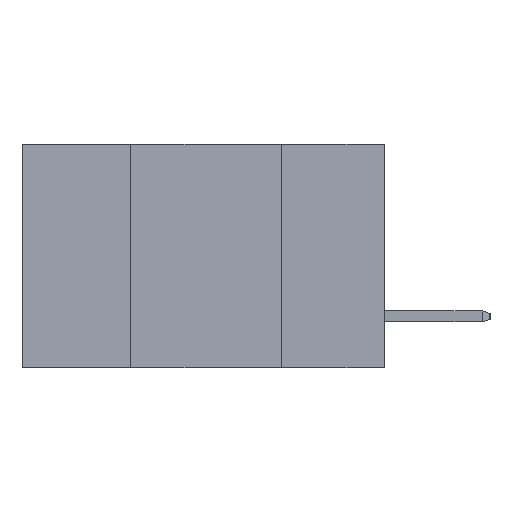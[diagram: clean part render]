
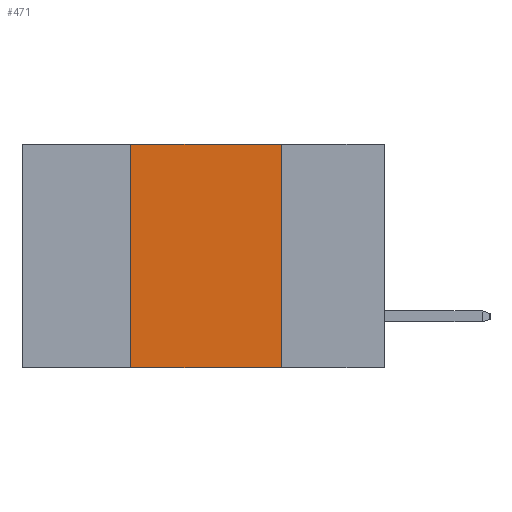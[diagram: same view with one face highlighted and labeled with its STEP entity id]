
A CAD part, left-side view. The second image highlights one B-rep face of the part: STEP entity #471.
In plain terms, the highlighted planar face has unit normal (-1, 0, 0).
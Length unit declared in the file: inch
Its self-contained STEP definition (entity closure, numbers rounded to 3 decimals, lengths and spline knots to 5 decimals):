
#471 = ADVANCED_FACE ( 'NONE', ( #11316 ), #24285, .F. ) ;
#1802 = DIRECTION ( 'NONE',  ( 0., 0., -1. ) ) ;
#3424 = CARTESIAN_POINT ( 'NONE',  ( 0., 0.42, -0.37 ) ) ;
#3860 = CARTESIAN_POINT ( 'NONE',  ( 0., 0.17, 0. ) ) ;
#3966 = DIRECTION ( 'NONE',  ( 0., -1., 0. ) ) ;
#5095 = LINE ( 'NONE', #14805, #22278 ) ;
#5142 = ORIENTED_EDGE ( 'NONE', *, *, #10030, .F. ) ;
#5227 = EDGE_CURVE ( 'NONE', #5744, #25978, #26703, .T. ) ;
#5744 = VERTEX_POINT ( 'NONE', #3860 ) ;
#6261 = CARTESIAN_POINT ( 'NONE',  ( 0., 0.6, 0. ) ) ;
#7250 = ORIENTED_EDGE ( 'NONE', *, *, #17440, .T. ) ;
#9217 = CARTESIAN_POINT ( 'NONE',  ( 0., 0.17, 0. ) ) ;
#10030 = EDGE_CURVE ( 'NONE', #25323, #18070, #23698, .T. ) ;
#10309 = DIRECTION ( 'NONE',  ( 0., -1., 0. ) ) ;
#10807 = CARTESIAN_POINT ( 'NONE',  ( 0., 0.6, 0. ) ) ;
#10934 = EDGE_CURVE ( 'NONE', #18070, #5744, #23215, .T. ) ;
#11316 = FACE_OUTER_BOUND ( 'NONE', #27347, .T. ) ;
#11336 = VECTOR ( 'NONE', #3966, 39.37008 ) ;
#11827 = VECTOR ( 'NONE', #21072, 39.37008 ) ;
#12388 = CARTESIAN_POINT ( 'NONE',  ( 0., 0.17, -0.37 ) ) ;
#13743 = DIRECTION ( 'NONE',  ( 0., 0., -1. ) ) ;
#14102 = DIRECTION ( 'NONE',  ( 1., 0., 0. ) ) ;
#14805 = CARTESIAN_POINT ( 'NONE',  ( 0., 0.6, -0.37 ) ) ;
#16592 = CARTESIAN_POINT ( 'NONE',  ( 0., 0.42, 0. ) ) ;
#17440 = EDGE_CURVE ( 'NONE', #25323, #25978, #5095, .T. ) ;
#18070 = VERTEX_POINT ( 'NONE', #18949 ) ;
#18949 = CARTESIAN_POINT ( 'NONE',  ( 0., 0.42, 0. ) ) ;
#19817 = ORIENTED_EDGE ( 'NONE', *, *, #5227, .F. ) ;
#20820 = VECTOR ( 'NONE', #13743, 39.37008 ) ;
#21072 = DIRECTION ( 'NONE',  ( 0., 0., 1. ) ) ;
#22278 = VECTOR ( 'NONE', #10309, 39.37008 ) ;
#23215 = LINE ( 'NONE', #6261, #11336 ) ;
#23698 = LINE ( 'NONE', #16592, #11827 ) ;
#24048 = ORIENTED_EDGE ( 'NONE', *, *, #10934, .F. ) ;
#24285 = PLANE ( 'NONE',  #27984 ) ;
#25323 = VERTEX_POINT ( 'NONE', #3424 ) ;
#25978 = VERTEX_POINT ( 'NONE', #12388 ) ;
#26703 = LINE ( 'NONE', #9217, #20820 ) ;
#27347 = EDGE_LOOP ( 'NONE', ( #19817, #24048, #5142, #7250 ) ) ;
#27984 = AXIS2_PLACEMENT_3D ( 'NONE', #10807, #14102, #1802 ) ;
